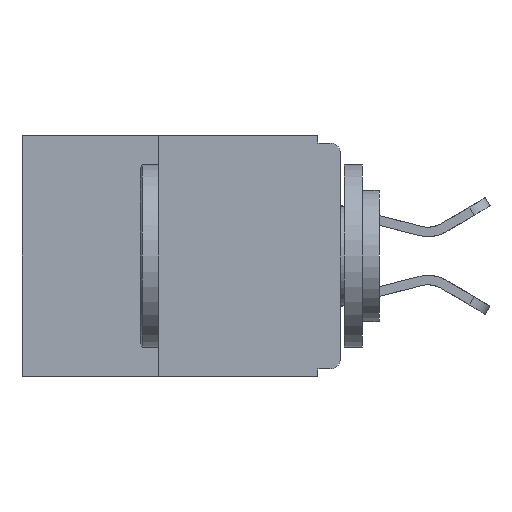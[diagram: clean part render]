
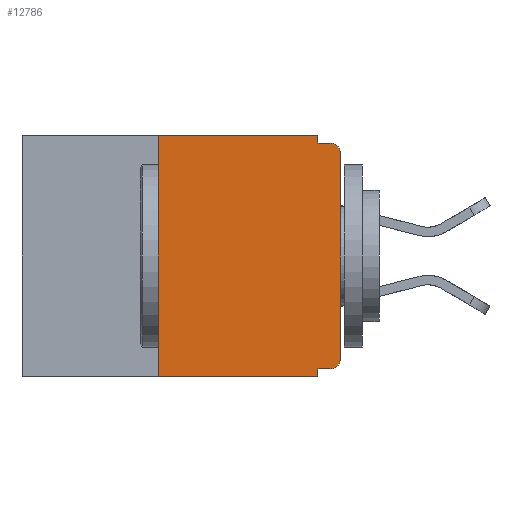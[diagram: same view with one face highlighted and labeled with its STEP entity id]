
A CAD part, left-side view. The second image highlights one B-rep face of the part: STEP entity #12786.
In plain terms, the highlighted planar face has unit normal (-1, 0, 0).
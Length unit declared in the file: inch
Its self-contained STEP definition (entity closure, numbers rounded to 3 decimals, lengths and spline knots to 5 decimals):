
#77 = EDGE_LOOP ( 'NONE', ( #16833, #5997, #19154, #102, #14135, #18425, #26835, #4504, #24968, #14200 ) ) ;
#98 = CARTESIAN_POINT ( 'NONE',  ( 0., 0.015, -0.32 ) ) ;
#102 = ORIENTED_EDGE ( 'NONE', *, *, #31058, .F. ) ;
#453 = CARTESIAN_POINT ( 'NONE',  ( 0., 0.031, -0.33 ) ) ;
#842 = CARTESIAN_POINT ( 'NONE',  ( 0., 0.031, -0.01 ) ) ;
#1821 = DIRECTION ( 'NONE',  ( 0., -1., 0. ) ) ;
#1878 = CARTESIAN_POINT ( 'NONE',  ( 0., 0., -0.305 ) ) ;
#2298 = VECTOR ( 'NONE', #18363, 39.37008 ) ;
#2430 = DIRECTION ( 'NONE',  ( 0., 0., -1. ) ) ;
#2457 = EDGE_CURVE ( 'NONE', #21981, #24277, #31280, .T. ) ;
#2674 = AXIS2_PLACEMENT_3D ( 'NONE', #31875, #17304, #2430 ) ;
#3112 = LINE ( 'NONE', #25639, #2298 ) ;
#3516 = EDGE_CURVE ( 'NONE', #21981, #16733, #20624, .T. ) ;
#3780 = VERTEX_POINT ( 'NONE', #7633 ) ;
#4234 = LINE ( 'NONE', #4324, #10058 ) ;
#4324 = CARTESIAN_POINT ( 'NONE',  ( 0., 0.031, 0. ) ) ;
#4504 = ORIENTED_EDGE ( 'NONE', *, *, #10766, .F. ) ;
#5233 = LINE ( 'NONE', #11755, #11075 ) ;
#5974 = PLANE ( 'NONE',  #14056 ) ;
#5997 = ORIENTED_EDGE ( 'NONE', *, *, #6416, .T. ) ;
#6416 = EDGE_CURVE ( 'NONE', #15042, #15521, #15814, .T. ) ;
#6812 = DIRECTION ( 'NONE',  ( 0., 0., -1. ) ) ;
#7633 = CARTESIAN_POINT ( 'NONE',  ( 0., 0.25, 0. ) ) ;
#8495 = DIRECTION ( 'NONE',  ( 0., 0., -1. ) ) ;
#9033 = CARTESIAN_POINT ( 'NONE',  ( 0., 0.031, 0. ) ) ;
#9151 = CARTESIAN_POINT ( 'NONE',  ( 0., 0.031, -0.33 ) ) ;
#9657 = DIRECTION ( 'NONE',  ( 0., 0., 1. ) ) ;
#9757 = CARTESIAN_POINT ( 'NONE',  ( 0., 0., -0.025 ) ) ;
#10058 = VECTOR ( 'NONE', #6812, 39.37008 ) ;
#10766 = EDGE_CURVE ( 'NONE', #24277, #15985, #30753, .T. ) ;
#10866 = CARTESIAN_POINT ( 'NONE',  ( 0., 0.437, -0.33 ) ) ;
#11075 = VECTOR ( 'NONE', #1821, 39.37008 ) ;
#11466 = FACE_OUTER_BOUND ( 'NONE', #77, .T. ) ;
#11755 = CARTESIAN_POINT ( 'NONE',  ( 0., 0.437, 0. ) ) ;
#11988 = CARTESIAN_POINT ( 'NONE',  ( 0., 0.015, -0.01 ) ) ;
#12023 = DIRECTION ( 'NONE',  ( 0., 0., 1. ) ) ;
#12786 = ADVANCED_FACE ( 'NONE', ( #11466 ), #5974, .F. ) ;
#13072 = EDGE_CURVE ( 'NONE', #27063, #3780, #21834, .T. ) ;
#13439 = AXIS2_PLACEMENT_3D ( 'NONE', #22528, #22501, #22408 ) ;
#14056 = AXIS2_PLACEMENT_3D ( 'NONE', #15852, #23284, #8495 ) ;
#14135 = ORIENTED_EDGE ( 'NONE', *, *, #25539, .F. ) ;
#14200 = ORIENTED_EDGE ( 'NONE', *, *, #3516, .T. ) ;
#15042 = VERTEX_POINT ( 'NONE', #9757 ) ;
#15500 = VECTOR ( 'NONE', #23263, 39.37008 ) ;
#15521 = VERTEX_POINT ( 'NONE', #11988 ) ;
#15814 = CIRCLE ( 'NONE', #2674, 0.015 ) ;
#15852 = CARTESIAN_POINT ( 'NONE',  ( 0., 0.437, 0. ) ) ;
#15985 = VERTEX_POINT ( 'NONE', #9151 ) ;
#16082 = VECTOR ( 'NONE', #12023, 39.37008 ) ;
#16733 = VERTEX_POINT ( 'NONE', #1878 ) ;
#16833 = ORIENTED_EDGE ( 'NONE', *, *, #23091, .T. ) ;
#17304 = DIRECTION ( 'NONE',  ( -1., 0., 0. ) ) ;
#18151 = CARTESIAN_POINT ( 'NONE',  ( 0., 0., -0.32 ) ) ;
#18363 = DIRECTION ( 'NONE',  ( 0., -1., 0. ) ) ;
#18425 = ORIENTED_EDGE ( 'NONE', *, *, #13072, .F. ) ;
#19154 = ORIENTED_EDGE ( 'NONE', *, *, #22179, .F. ) ;
#20624 = CIRCLE ( 'NONE', #13439, 0.015 ) ;
#21453 = DIRECTION ( 'NONE',  ( 0., 1., 0. ) ) ;
#21834 = LINE ( 'NONE', #24290, #16082 ) ;
#21940 = CARTESIAN_POINT ( 'NONE',  ( 0., 0., 0. ) ) ;
#21981 = VERTEX_POINT ( 'NONE', #98 ) ;
#22017 = LINE ( 'NONE', #10866, #15500 ) ;
#22179 = EDGE_CURVE ( 'NONE', #25306, #15521, #3112, .T. ) ;
#22408 = DIRECTION ( 'NONE',  ( 0., 0., -1. ) ) ;
#22501 = DIRECTION ( 'NONE',  ( -1., 0., 0. ) ) ;
#22528 = CARTESIAN_POINT ( 'NONE',  ( 0., 0.015, -0.305 ) ) ;
#23091 = EDGE_CURVE ( 'NONE', #16733, #15042, #26217, .T. ) ;
#23263 = DIRECTION ( 'NONE',  ( 0., -1., 0. ) ) ;
#23284 = DIRECTION ( 'NONE',  ( 1., 0., 0. ) ) ;
#23554 = VECTOR ( 'NONE', #25253, 39.37008 ) ;
#24277 = VERTEX_POINT ( 'NONE', #26327 ) ;
#24290 = CARTESIAN_POINT ( 'NONE',  ( 0., 0.25, -0.33 ) ) ;
#24968 = ORIENTED_EDGE ( 'NONE', *, *, #2457, .F. ) ;
#25253 = DIRECTION ( 'NONE',  ( 0., 0., -1. ) ) ;
#25306 = VERTEX_POINT ( 'NONE', #842 ) ;
#25452 = VECTOR ( 'NONE', #9657, 39.37008 ) ;
#25539 = EDGE_CURVE ( 'NONE', #3780, #30364, #5233, .T. ) ;
#25608 = VECTOR ( 'NONE', #21453, 39.37008 ) ;
#25639 = CARTESIAN_POINT ( 'NONE',  ( 0., 0., -0.01 ) ) ;
#26217 = LINE ( 'NONE', #21940, #25452 ) ;
#26327 = CARTESIAN_POINT ( 'NONE',  ( 0., 0.031, -0.32 ) ) ;
#26835 = ORIENTED_EDGE ( 'NONE', *, *, #30839, .T. ) ;
#27063 = VERTEX_POINT ( 'NONE', #28121 ) ;
#28121 = CARTESIAN_POINT ( 'NONE',  ( 0., 0.25, -0.33 ) ) ;
#30364 = VERTEX_POINT ( 'NONE', #9033 ) ;
#30753 = LINE ( 'NONE', #453, #23554 ) ;
#30839 = EDGE_CURVE ( 'NONE', #27063, #15985, #22017, .T. ) ;
#31058 = EDGE_CURVE ( 'NONE', #30364, #25306, #4234, .T. ) ;
#31280 = LINE ( 'NONE', #18151, #25608 ) ;
#31875 = CARTESIAN_POINT ( 'NONE',  ( 0., 0.015, -0.025 ) ) ;
